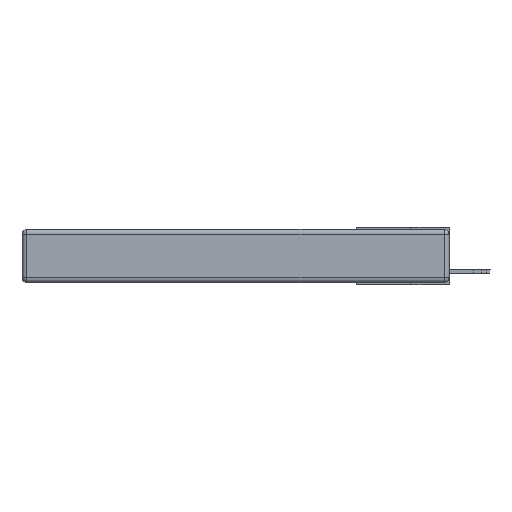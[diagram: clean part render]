
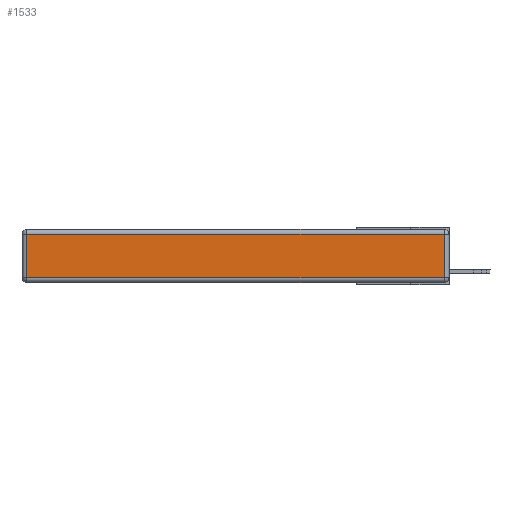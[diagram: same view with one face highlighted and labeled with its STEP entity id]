
A CAD part, left-side view. The second image highlights one B-rep face of the part: STEP entity #1533.
In plain terms, the highlighted planar face has unit normal (-1, 0, 0).
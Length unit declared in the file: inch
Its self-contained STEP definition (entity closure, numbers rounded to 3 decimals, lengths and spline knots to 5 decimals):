
#421 = CARTESIAN_POINT ( 'NONE',  ( 0., 0., -0.343 ) ) ;
#471 = DIRECTION ( 'NONE',  ( 0., 0., 1. ) ) ;
#1023 = AXIS2_PLACEMENT_3D ( 'NONE', #421, #10319, #471 ) ;
#1088 = ORIENTED_EDGE ( 'NONE', *, *, #10077, .T. ) ;
#1326 = CARTESIAN_POINT ( 'NONE',  ( 0., 2.72, -0.343 ) ) ;
#1533 = ADVANCED_FACE ( 'NONE', ( #8221 ), #8285, .T. ) ;
#2118 = ORIENTED_EDGE ( 'NONE', *, *, #4894, .T. ) ;
#2440 = ORIENTED_EDGE ( 'NONE', *, *, #4491, .T. ) ;
#2481 = DIRECTION ( 'NONE',  ( 0., 0., -1. ) ) ;
#2936 = VECTOR ( 'NONE', #10190, 39.37008 ) ;
#3064 = DIRECTION ( 'NONE',  ( 0., -1., 0. ) ) ;
#3074 = VERTEX_POINT ( 'NONE', #10751 ) ;
#3211 = CARTESIAN_POINT ( 'NONE',  ( 0., 0., -0.313 ) ) ;
#4491 = EDGE_CURVE ( 'NONE', #13347, #3074, #4506, .T. ) ;
#4506 = LINE ( 'NONE', #6863, #2936 ) ;
#4751 = LINE ( 'NONE', #3211, #11762 ) ;
#4894 = EDGE_CURVE ( 'NONE', #3074, #10577, #12396, .T. ) ;
#5140 = CARTESIAN_POINT ( 'NONE',  ( 0., 0.03, -0.313 ) ) ;
#6358 = VERTEX_POINT ( 'NONE', #5140 ) ;
#6863 = CARTESIAN_POINT ( 'NONE',  ( 0., 2.75, -0.03 ) ) ;
#6927 = VECTOR ( 'NONE', #2481, 39.37008 ) ;
#7161 = VECTOR ( 'NONE', #12487, 39.37008 ) ;
#8221 = FACE_OUTER_BOUND ( 'NONE', #13200, .T. ) ;
#8225 = CARTESIAN_POINT ( 'NONE',  ( 0., 0.03, -0.343 ) ) ;
#8285 = PLANE ( 'NONE',  #1023 ) ;
#9798 = EDGE_CURVE ( 'NONE', #6358, #13347, #13823, .T. ) ;
#10028 = CARTESIAN_POINT ( 'NONE',  ( 0., 2.72, -0.313 ) ) ;
#10077 = EDGE_CURVE ( 'NONE', #10577, #6358, #4751, .T. ) ;
#10190 = DIRECTION ( 'NONE',  ( 0., 1., 0. ) ) ;
#10319 = DIRECTION ( 'NONE',  ( -1., 0., 0. ) ) ;
#10478 = CARTESIAN_POINT ( 'NONE',  ( 0., 0.03, -0.03 ) ) ;
#10577 = VERTEX_POINT ( 'NONE', #10028 ) ;
#10751 = CARTESIAN_POINT ( 'NONE',  ( 0., 2.72, -0.03 ) ) ;
#11762 = VECTOR ( 'NONE', #3064, 39.37008 ) ;
#12120 = ORIENTED_EDGE ( 'NONE', *, *, #9798, .T. ) ;
#12396 = LINE ( 'NONE', #1326, #6927 ) ;
#12487 = DIRECTION ( 'NONE',  ( 0., 0., 1. ) ) ;
#13200 = EDGE_LOOP ( 'NONE', ( #1088, #12120, #2440, #2118 ) ) ;
#13347 = VERTEX_POINT ( 'NONE', #10478 ) ;
#13823 = LINE ( 'NONE', #8225, #7161 ) ;
